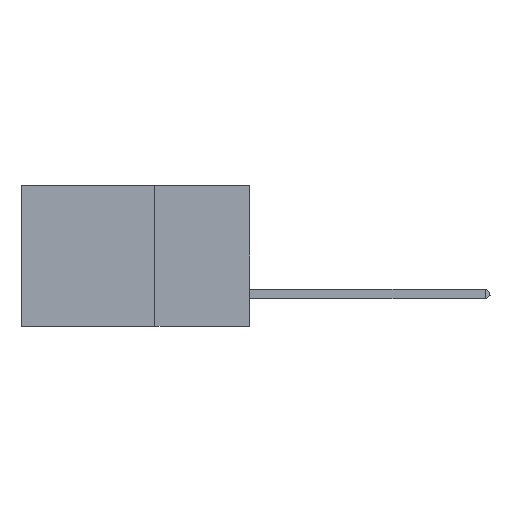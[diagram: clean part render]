
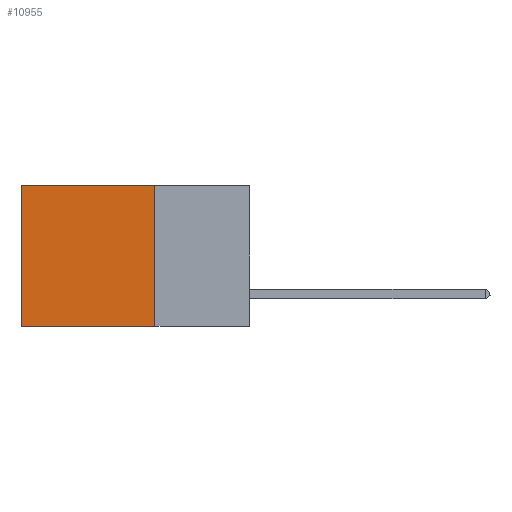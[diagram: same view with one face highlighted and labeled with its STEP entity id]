
A CAD part, left-side view. The second image highlights one B-rep face of the part: STEP entity #10955.
In plain terms, the highlighted planar face has unit normal (-1, 0, 0).
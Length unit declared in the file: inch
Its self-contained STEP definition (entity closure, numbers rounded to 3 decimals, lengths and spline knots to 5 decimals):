
#458 = LINE ( 'NONE', #9717, #10524 ) ;
#2333 = VERTEX_POINT ( 'NONE', #7085 ) ;
#2844 = CARTESIAN_POINT ( 'NONE',  ( 0.2875, 0.25, 0. ) ) ;
#3097 = EDGE_CURVE ( 'NONE', #6629, #2333, #8060, .T. ) ;
#3147 = CARTESIAN_POINT ( 'NONE',  ( 0.2875, 0.6, 0. ) ) ;
#3543 = DIRECTION ( 'NONE',  ( 0., 0., -1. ) ) ;
#4116 = ORIENTED_EDGE ( 'NONE', *, *, #10560, .F. ) ;
#4397 = DIRECTION ( 'NONE',  ( 1., 0., 0. ) ) ;
#4748 = VECTOR ( 'NONE', #3543, 39.37008 ) ;
#6629 = VERTEX_POINT ( 'NONE', #16696 ) ;
#6842 = VECTOR ( 'NONE', #16164, 39.37008 ) ;
#7085 = CARTESIAN_POINT ( 'NONE',  ( 0.2875, 0.6, -0.37 ) ) ;
#7309 = ORIENTED_EDGE ( 'NONE', *, *, #3097, .T. ) ;
#8060 = LINE ( 'NONE', #3147, #4748 ) ;
#8080 = VECTOR ( 'NONE', #10205, 39.37008 ) ;
#8305 = EDGE_CURVE ( 'NONE', #10457, #12662, #12159, .T. ) ;
#9717 = CARTESIAN_POINT ( 'NONE',  ( 0.2875, 0.25, 0. ) ) ;
#10205 = DIRECTION ( 'NONE',  ( 0., 0., -1. ) ) ;
#10387 = EDGE_LOOP ( 'NONE', ( #7309, #4116, #17017, #13758 ) ) ;
#10434 = DIRECTION ( 'NONE',  ( 0., 0., -1. ) ) ;
#10457 = VERTEX_POINT ( 'NONE', #12195 ) ;
#10524 = VECTOR ( 'NONE', #14339, 39.37008 ) ;
#10560 = EDGE_CURVE ( 'NONE', #12662, #2333, #10882, .T. ) ;
#10882 = LINE ( 'NONE', #17574, #6842 ) ;
#10955 = ADVANCED_FACE ( 'NONE', ( #14947 ), #17651, .F. ) ;
#12159 = LINE ( 'NONE', #17623, #8080 ) ;
#12195 = CARTESIAN_POINT ( 'NONE',  ( 0.2875, 0.25, 0. ) ) ;
#12662 = VERTEX_POINT ( 'NONE', #19454 ) ;
#13758 = ORIENTED_EDGE ( 'NONE', *, *, #15732, .T. ) ;
#14339 = DIRECTION ( 'NONE',  ( 0., 1., 0. ) ) ;
#14947 = FACE_OUTER_BOUND ( 'NONE', #10387, .T. ) ;
#15732 = EDGE_CURVE ( 'NONE', #10457, #6629, #458, .T. ) ;
#16164 = DIRECTION ( 'NONE',  ( 0., 1., 0. ) ) ;
#16696 = CARTESIAN_POINT ( 'NONE',  ( 0.2875, 0.6, 0. ) ) ;
#17017 = ORIENTED_EDGE ( 'NONE', *, *, #8305, .F. ) ;
#17574 = CARTESIAN_POINT ( 'NONE',  ( 0.2875, 0.25, -0.37 ) ) ;
#17623 = CARTESIAN_POINT ( 'NONE',  ( 0.2875, 0.25, 0. ) ) ;
#17651 = PLANE ( 'NONE',  #18824 ) ;
#18824 = AXIS2_PLACEMENT_3D ( 'NONE', #2844, #4397, #10434 ) ;
#19454 = CARTESIAN_POINT ( 'NONE',  ( 0.2875, 0.25, -0.37 ) ) ;
